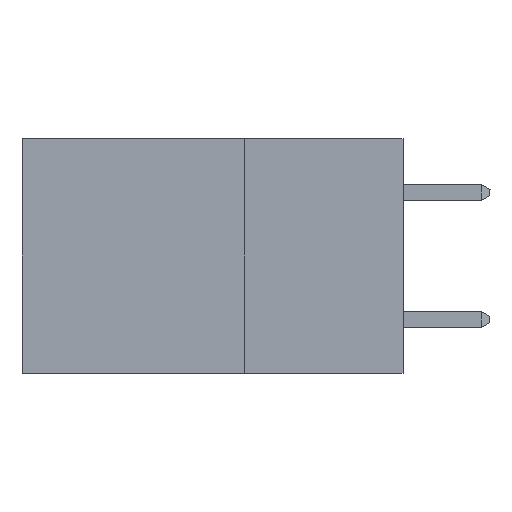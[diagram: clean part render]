
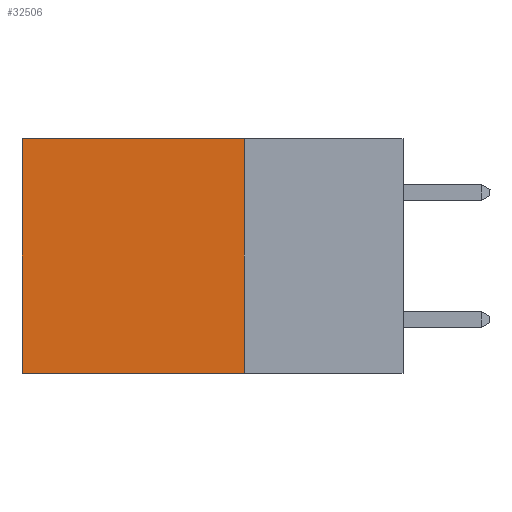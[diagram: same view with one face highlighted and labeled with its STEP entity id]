
A CAD part, left-side view. The second image highlights one B-rep face of the part: STEP entity #32506.
In plain terms, the highlighted planar face has unit normal (-1, 0, 0).
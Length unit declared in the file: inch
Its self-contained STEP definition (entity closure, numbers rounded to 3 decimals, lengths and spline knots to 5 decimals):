
#120 = PLANE ( 'NONE',  #28627 ) ;
#973 = CARTESIAN_POINT ( 'NONE',  ( 0.2875, 0.25, 0. ) ) ;
#2278 = DIRECTION ( 'NONE',  ( 0., 0., -1. ) ) ;
#3814 = CARTESIAN_POINT ( 'NONE',  ( 0.2875, 0.25, 0. ) ) ;
#5066 = LINE ( 'NONE', #24458, #33092 ) ;
#6567 = EDGE_CURVE ( 'NONE', #37864, #19865, #39313, .T. ) ;
#7496 = DIRECTION ( 'NONE',  ( 1., 0., 0. ) ) ;
#10309 = EDGE_LOOP ( 'NONE', ( #16968, #36959, #11492, #19661 ) ) ;
#11492 = ORIENTED_EDGE ( 'NONE', *, *, #38215, .F. ) ;
#11750 = LINE ( 'NONE', #14426, #31207 ) ;
#12328 = EDGE_CURVE ( 'NONE', #20768, #37864, #19526, .T. ) ;
#14426 = CARTESIAN_POINT ( 'NONE',  ( 0.2875, 0.25, 0. ) ) ;
#16767 = FACE_OUTER_BOUND ( 'NONE', #10309, .T. ) ;
#16968 = ORIENTED_EDGE ( 'NONE', *, *, #6567, .T. ) ;
#18731 = CARTESIAN_POINT ( 'NONE',  ( 0.2875, 0.25, 0. ) ) ;
#19526 = LINE ( 'NONE', #973, #46210 ) ;
#19661 = ORIENTED_EDGE ( 'NONE', *, *, #12328, .T. ) ;
#19865 = VERTEX_POINT ( 'NONE', #28747 ) ;
#20768 = VERTEX_POINT ( 'NONE', #18731 ) ;
#24458 = CARTESIAN_POINT ( 'NONE',  ( 0.2875, 0.25, -0.37 ) ) ;
#26853 = VERTEX_POINT ( 'NONE', #38927 ) ;
#28627 = AXIS2_PLACEMENT_3D ( 'NONE', #3814, #7496, #33061 ) ;
#28747 = CARTESIAN_POINT ( 'NONE',  ( 0.2875, 0.6, -0.37 ) ) ;
#31207 = VECTOR ( 'NONE', #39886, 39.37008 ) ;
#32506 = ADVANCED_FACE ( 'NONE', ( #16767 ), #120, .F. ) ;
#33061 = DIRECTION ( 'NONE',  ( 0., 0., -1. ) ) ;
#33092 = VECTOR ( 'NONE', #35317, 39.37008 ) ;
#35099 = CARTESIAN_POINT ( 'NONE',  ( 0.2875, 0.6, 0. ) ) ;
#35317 = DIRECTION ( 'NONE',  ( 0., 1., 0. ) ) ;
#36959 = ORIENTED_EDGE ( 'NONE', *, *, #44494, .F. ) ;
#37602 = DIRECTION ( 'NONE',  ( 0., 1., 0. ) ) ;
#37864 = VERTEX_POINT ( 'NONE', #39205 ) ;
#38215 = EDGE_CURVE ( 'NONE', #20768, #26853, #11750, .T. ) ;
#38927 = CARTESIAN_POINT ( 'NONE',  ( 0.2875, 0.25, -0.37 ) ) ;
#39205 = CARTESIAN_POINT ( 'NONE',  ( 0.2875, 0.6, 0. ) ) ;
#39313 = LINE ( 'NONE', #35099, #40419 ) ;
#39886 = DIRECTION ( 'NONE',  ( 0., 0., -1. ) ) ;
#40419 = VECTOR ( 'NONE', #2278, 39.37008 ) ;
#44494 = EDGE_CURVE ( 'NONE', #26853, #19865, #5066, .T. ) ;
#46210 = VECTOR ( 'NONE', #37602, 39.37008 ) ;
